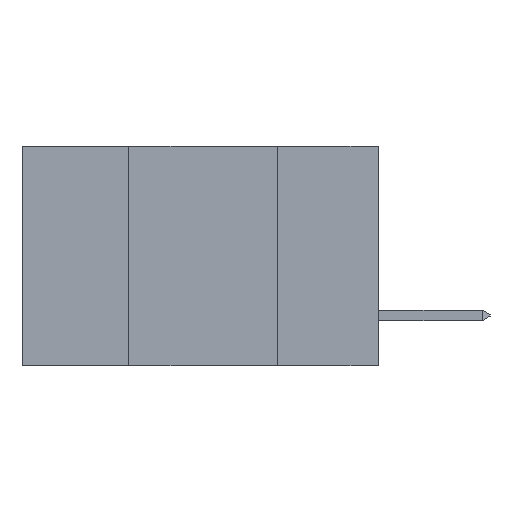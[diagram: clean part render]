
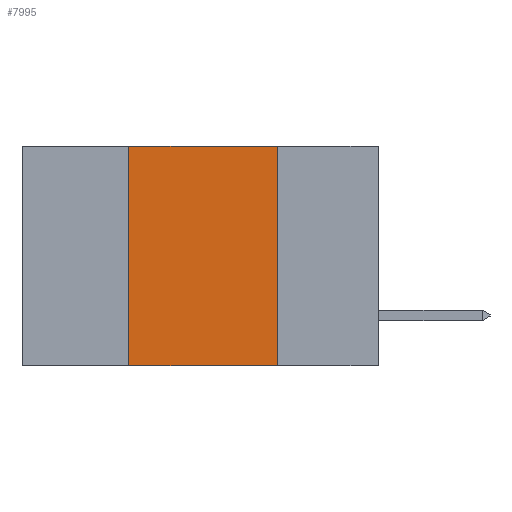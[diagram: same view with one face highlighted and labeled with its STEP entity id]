
A CAD part, left-side view. The second image highlights one B-rep face of the part: STEP entity #7995.
In plain terms, the highlighted planar face has unit normal (-1, 0, 0).
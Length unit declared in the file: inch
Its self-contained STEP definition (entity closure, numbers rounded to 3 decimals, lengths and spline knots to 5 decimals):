
#13 = DIRECTION ( 'NONE',  ( 0., 0., 1. ) ) ;
#111 = AXIS2_PLACEMENT_3D ( 'NONE', #8793, #9818, #3593 ) ;
#1002 = CARTESIAN_POINT ( 'NONE',  ( 0., 0.42, -0.37 ) ) ;
#1133 = CARTESIAN_POINT ( 'NONE',  ( 0., 0.6, -0.37 ) ) ;
#1185 = ORIENTED_EDGE ( 'NONE', *, *, #1523, .F. ) ;
#1195 = DIRECTION ( 'NONE',  ( 0., -1., 0. ) ) ;
#1247 = EDGE_CURVE ( 'NONE', #8815, #4079, #5419, .T. ) ;
#1523 = EDGE_CURVE ( 'NONE', #8854, #6737, #12225, .T. ) ;
#1540 = PLANE ( 'NONE',  #111 ) ;
#2327 = VECTOR ( 'NONE', #11953, 39.37008 ) ;
#2637 = CARTESIAN_POINT ( 'NONE',  ( 0., 0.17, 0. ) ) ;
#3161 = DIRECTION ( 'NONE',  ( 0., 0., -1. ) ) ;
#3222 = LINE ( 'NONE', #9388, #8757 ) ;
#3330 = EDGE_LOOP ( 'NONE', ( #7195, #1185, #3941, #8124 ) ) ;
#3593 = DIRECTION ( 'NONE',  ( 0., 0., -1. ) ) ;
#3625 = CARTESIAN_POINT ( 'NONE',  ( 0., 0.6, 0. ) ) ;
#3941 = ORIENTED_EDGE ( 'NONE', *, *, #9850, .F. ) ;
#4079 = VERTEX_POINT ( 'NONE', #6054 ) ;
#5419 = LINE ( 'NONE', #1133, #2327 ) ;
#5463 = VECTOR ( 'NONE', #13, 39.37008 ) ;
#6054 = CARTESIAN_POINT ( 'NONE',  ( 0., 0.17, -0.37 ) ) ;
#6737 = VERTEX_POINT ( 'NONE', #2637 ) ;
#7043 = VECTOR ( 'NONE', #1195, 39.37008 ) ;
#7195 = ORIENTED_EDGE ( 'NONE', *, *, #7721, .F. ) ;
#7721 = EDGE_CURVE ( 'NONE', #6737, #4079, #3222, .T. ) ;
#7995 = ADVANCED_FACE ( 'NONE', ( #10703 ), #1540, .F. ) ;
#8124 = ORIENTED_EDGE ( 'NONE', *, *, #1247, .T. ) ;
#8222 = LINE ( 'NONE', #8898, #5463 ) ;
#8757 = VECTOR ( 'NONE', #3161, 39.37008 ) ;
#8793 = CARTESIAN_POINT ( 'NONE',  ( 0., 0.6, 0. ) ) ;
#8815 = VERTEX_POINT ( 'NONE', #1002 ) ;
#8854 = VERTEX_POINT ( 'NONE', #9404 ) ;
#8898 = CARTESIAN_POINT ( 'NONE',  ( 0., 0.42, -0.37 ) ) ;
#9388 = CARTESIAN_POINT ( 'NONE',  ( 0., 0.17, -0.37 ) ) ;
#9404 = CARTESIAN_POINT ( 'NONE',  ( 0., 0.42, 0. ) ) ;
#9818 = DIRECTION ( 'NONE',  ( 1., 0., 0. ) ) ;
#9850 = EDGE_CURVE ( 'NONE', #8815, #8854, #8222, .T. ) ;
#10703 = FACE_OUTER_BOUND ( 'NONE', #3330, .T. ) ;
#11953 = DIRECTION ( 'NONE',  ( 0., -1., 0. ) ) ;
#12225 = LINE ( 'NONE', #3625, #7043 ) ;
